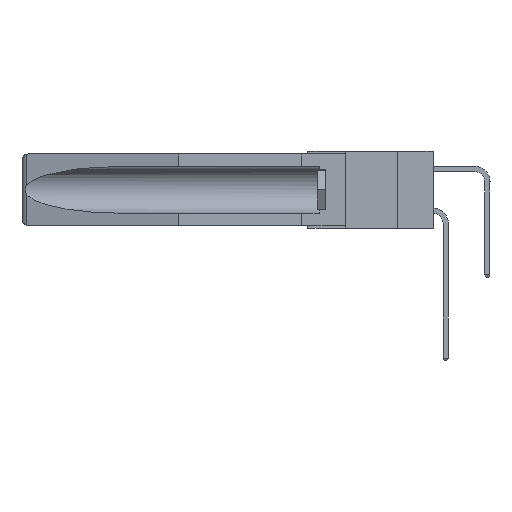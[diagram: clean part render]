
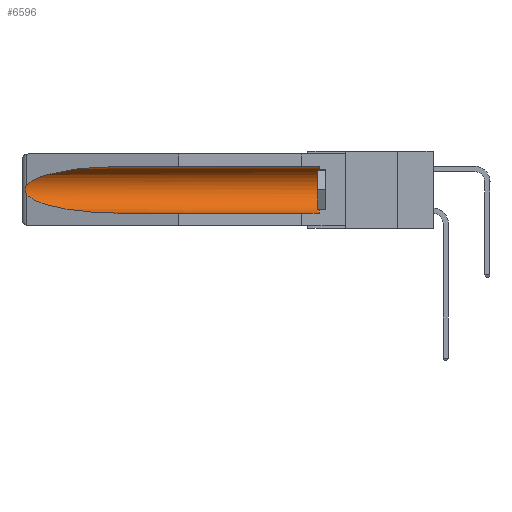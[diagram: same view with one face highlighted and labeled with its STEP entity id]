
A CAD part, left-side view. The second image highlights one B-rep face of the part: STEP entity #6596.
In plain terms, the highlighted cylindrical face has radius 2.857 mm (diameter 5.715 mm), a partial arc.
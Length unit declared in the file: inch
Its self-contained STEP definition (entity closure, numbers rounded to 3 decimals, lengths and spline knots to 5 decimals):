
#233 = CARTESIAN_POINT ( 'NONE',  ( 0.26537, 1.52718, -0.19328 ) ) ;
#961 = CARTESIAN_POINT ( 'NONE',  ( 0.26597, 1.52961, -0.15275 ) ) ;
#1258 = VERTEX_POINT ( 'NONE', #9808 ) ;
#1319 = VECTOR ( 'NONE', #4779, 39.37008 ) ;
#1594 = EDGE_CURVE ( 'NONE', #8886, #1258, #21630, .T. ) ;
#2006 = CYLINDRICAL_SURFACE ( 'NONE', #19142, 0.1125 ) ;
#3292 = CARTESIAN_POINT ( 'NONE',  ( 0.26597, 1.5296, -0.19026 ) ) ;
#4341 = ORIENTED_EDGE ( 'NONE', *, *, #13510, .T. ) ;
#4404 = ORIENTED_EDGE ( 'NONE', *, *, #16384, .T. ) ;
#4779 = DIRECTION ( 'NONE',  ( 0., 1., 0. ) ) ;
#5427 = LINE ( 'NONE', #23783, #11053 ) ;
#6182 = CARTESIAN_POINT ( 'NONE',  ( 0.155, 1.07973, -0.059 ) ) ;
#6272 = CARTESIAN_POINT ( 'NONE',  ( 0.26537, 1.52718, -0.14972 ) ) ;
#6346 = B_SPLINE_CURVE_WITH_KNOTS ( 'NONE', 3,
 ( #22251, #961, #14686, #16631, #20809, #12855, #20716, #9182, #3292, #22535 ),
 .UNSPECIFIED., .F., .F.,
 ( 4, 2, 2, 2, 4 ),
 ( 0., 0.00029, 0.00058, 0.00087, 0.00117 ),
 .UNSPECIFIED. ) ;
#6414 = CARTESIAN_POINT ( 'NONE',  ( 0.155, 1.07973, -0.284 ) ) ;
#6552 = ORIENTED_EDGE ( 'NONE', *, *, #1594, .T. ) ;
#6596 = ADVANCED_FACE ( 'NONE', ( #20244 ), #2006, .F. ) ;
#6754 = VERTEX_POINT ( 'NONE', #20365 ) ;
#7012 = DIRECTION ( 'NONE',  ( 0., 1., 0. ) ) ;
#7463 = VERTEX_POINT ( 'NONE', #11039 ) ;
#7895 = CARTESIAN_POINT ( 'NONE',  ( 0.25451, 1.48313, -0.24835 ) ) ;
#8331 = ORIENTED_EDGE ( 'NONE', *, *, #15910, .T. ) ;
#8732 = VERTEX_POINT ( 'NONE', #233 ) ;
#8886 = VERTEX_POINT ( 'NONE', #16809 ) ;
#9013 = CARTESIAN_POINT ( 'NONE',  ( 0.155, 0.126, -0.1715 ) ) ;
#9182 = CARTESIAN_POINT ( 'NONE',  ( 0.26655, 1.53094, -0.18657 ) ) ;
#9184 = EDGE_CURVE ( 'NONE', #8886, #13968, #17773, .T. ) ;
#9193 =( BOUNDED_CURVE ( )  B_SPLINE_CURVE ( 3, ( #15384, #7895, #11804, #17427 ),
 .UNSPECIFIED., .F., .F. ) 
 B_SPLINE_CURVE_WITH_KNOTS ( ( 4, 4 ),
 ( 0.1948, 1.5708 ),
 .UNSPECIFIED. ) 
 CURVE ( )  GEOMETRIC_REPRESENTATION_ITEM ( )  RATIONAL_B_SPLINE_CURVE ( ( 1., 0.848, 0.848, 1. ) ) 
 REPRESENTATION_ITEM ( '' )  );
#9808 = CARTESIAN_POINT ( 'NONE',  ( 0.155, 0.126, -0.059 ) ) ;
#11039 = CARTESIAN_POINT ( 'NONE',  ( 0.155, 1.07973, -0.059 ) ) ;
#11053 = VECTOR ( 'NONE', #7012, 39.37008 ) ;
#11499 =( BOUNDED_CURVE ( )  B_SPLINE_CURVE ( 3, ( #6182, #19557, #17697, #6272 ),
 .UNSPECIFIED., .F., .F. ) 
 B_SPLINE_CURVE_WITH_KNOTS ( ( 4, 4 ),
 ( 4.71239, 6.08839 ),
 .UNSPECIFIED. ) 
 CURVE ( )  GEOMETRIC_REPRESENTATION_ITEM ( )  RATIONAL_B_SPLINE_CURVE ( ( 1., 0.848, 0.848, 1. ) ) 
 REPRESENTATION_ITEM ( '' )  );
#11804 = CARTESIAN_POINT ( 'NONE',  ( 0.21114, 1.30732, -0.284 ) ) ;
#11818 = CARTESIAN_POINT ( 'NONE',  ( 0.155, -0.30754, -0.1715 ) ) ;
#11866 = ORIENTED_EDGE ( 'NONE', *, *, #16717, .T. ) ;
#12855 = CARTESIAN_POINT ( 'NONE',  ( 0.2675, 1.53308, -0.17534 ) ) ;
#13012 = DIRECTION ( 'NONE',  ( 0., 0., 1. ) ) ;
#13510 = EDGE_CURVE ( 'NONE', #7463, #6754, #11499, .T. ) ;
#13968 = VERTEX_POINT ( 'NONE', #6414 ) ;
#13997 = DIRECTION ( 'NONE',  ( 0., 1., 0. ) ) ;
#14686 = CARTESIAN_POINT ( 'NONE',  ( 0.26654, 1.53092, -0.15636 ) ) ;
#15384 = CARTESIAN_POINT ( 'NONE',  ( 0.26537, 1.52718, -0.19328 ) ) ;
#15910 = EDGE_CURVE ( 'NONE', #6754, #8732, #6346, .T. ) ;
#16384 = EDGE_CURVE ( 'NONE', #1258, #7463, #5427, .T. ) ;
#16631 = CARTESIAN_POINT ( 'NONE',  ( 0.2673, 1.5327, -0.16383 ) ) ;
#16717 = EDGE_CURVE ( 'NONE', #8732, #13968, #9193, .T. ) ;
#16809 = CARTESIAN_POINT ( 'NONE',  ( 0.155, 0.126, -0.284 ) ) ;
#17427 = CARTESIAN_POINT ( 'NONE',  ( 0.155, 1.07973, -0.284 ) ) ;
#17613 = DIRECTION ( 'NONE',  ( 0., 0., 1. ) ) ;
#17697 = CARTESIAN_POINT ( 'NONE',  ( 0.25451, 1.48313, -0.09465 ) ) ;
#17773 = LINE ( 'NONE', #20046, #1319 ) ;
#19142 = AXIS2_PLACEMENT_3D ( 'NONE', #11818, #13997, #17613 ) ;
#19557 = CARTESIAN_POINT ( 'NONE',  ( 0.21114, 1.30732, -0.059 ) ) ;
#20046 = CARTESIAN_POINT ( 'NONE',  ( 0.155, -0.30754, -0.284 ) ) ;
#20089 = EDGE_LOOP ( 'NONE', ( #4341, #8331, #11866, #23949, #6552, #4404 ) ) ;
#20244 = FACE_OUTER_BOUND ( 'NONE', #20089, .T. ) ;
#20365 = CARTESIAN_POINT ( 'NONE',  ( 0.26537, 1.52718, -0.14972 ) ) ;
#20716 = CARTESIAN_POINT ( 'NONE',  ( 0.2673, 1.53269, -0.17917 ) ) ;
#20809 = CARTESIAN_POINT ( 'NONE',  ( 0.2675, 1.53308, -0.16763 ) ) ;
#20946 = AXIS2_PLACEMENT_3D ( 'NONE', #9013, #24364, #13012 ) ;
#21630 = CIRCLE ( 'NONE', #20946, 0.1125 ) ;
#22251 = CARTESIAN_POINT ( 'NONE',  ( 0.26537, 1.52718, -0.14972 ) ) ;
#22535 = CARTESIAN_POINT ( 'NONE',  ( 0.26537, 1.52718, -0.19328 ) ) ;
#23783 = CARTESIAN_POINT ( 'NONE',  ( 0.155, -0.30754, -0.059 ) ) ;
#23949 = ORIENTED_EDGE ( 'NONE', *, *, #9184, .F. ) ;
#24364 = DIRECTION ( 'NONE',  ( 0., -1., 0. ) ) ;
